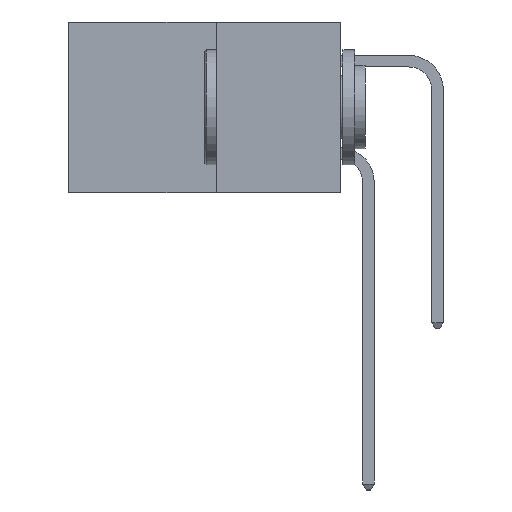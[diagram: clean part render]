
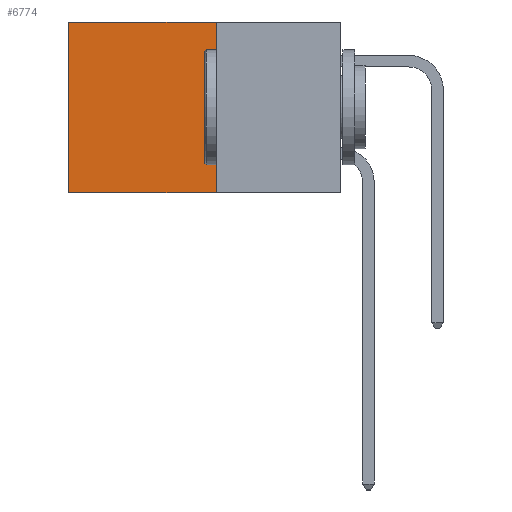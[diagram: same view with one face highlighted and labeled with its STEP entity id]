
A CAD part, left-side view. The second image highlights one B-rep face of the part: STEP entity #6774.
In plain terms, the highlighted planar face has unit normal (-1, 0, 0).
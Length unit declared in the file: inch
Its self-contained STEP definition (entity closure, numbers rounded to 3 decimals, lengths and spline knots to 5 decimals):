
#149 = VERTEX_POINT ( 'NONE', #4428 ) ;
#946 = EDGE_CURVE ( 'NONE', #6212, #1272, #7006, .T. ) ;
#1272 = VERTEX_POINT ( 'NONE', #6897 ) ;
#1538 = DIRECTION ( 'NONE',  ( 1., 0., 0. ) ) ;
#1558 = EDGE_LOOP ( 'NONE', ( #9436, #2102, #3152, #6438 ) ) ;
#2102 = ORIENTED_EDGE ( 'NONE', *, *, #9249, .F. ) ;
#2334 = EDGE_CURVE ( 'NONE', #6212, #7395, #4607, .T. ) ;
#2487 = VECTOR ( 'NONE', #5780, 39.37008 ) ;
#2665 = CARTESIAN_POINT ( 'NONE',  ( 0.277, 0.27, -0.37 ) ) ;
#3152 = ORIENTED_EDGE ( 'NONE', *, *, #946, .F. ) ;
#3175 = CARTESIAN_POINT ( 'NONE',  ( 0.277, 0.59, 0. ) ) ;
#3293 = AXIS2_PLACEMENT_3D ( 'NONE', #6301, #1538, #7115 ) ;
#3667 = LINE ( 'NONE', #8881, #7391 ) ;
#4302 = CARTESIAN_POINT ( 'NONE',  ( 0.277, 0.27, -0.37 ) ) ;
#4428 = CARTESIAN_POINT ( 'NONE',  ( 0.277, 0.59, -0.37 ) ) ;
#4607 = LINE ( 'NONE', #6411, #2487 ) ;
#4638 = VECTOR ( 'NONE', #9925, 39.37008 ) ;
#4718 = CARTESIAN_POINT ( 'NONE',  ( 0.277, 0.27, 0. ) ) ;
#5780 = DIRECTION ( 'NONE',  ( 0., 1., 0. ) ) ;
#6212 = VERTEX_POINT ( 'NONE', #4718 ) ;
#6301 = CARTESIAN_POINT ( 'NONE',  ( 0.277, 0.27, -0.37 ) ) ;
#6411 = CARTESIAN_POINT ( 'NONE',  ( 0.277, 0.27, 0. ) ) ;
#6438 = ORIENTED_EDGE ( 'NONE', *, *, #2334, .T. ) ;
#6458 = DIRECTION ( 'NONE',  ( 0., 0., -1. ) ) ;
#6774 = ADVANCED_FACE ( 'NONE', ( #9817 ), #9508, .F. ) ;
#6897 = CARTESIAN_POINT ( 'NONE',  ( 0.277, 0.27, -0.37 ) ) ;
#7006 = LINE ( 'NONE', #2665, #4638 ) ;
#7115 = DIRECTION ( 'NONE',  ( 0., 0., -1. ) ) ;
#7391 = VECTOR ( 'NONE', #6458, 39.37008 ) ;
#7395 = VERTEX_POINT ( 'NONE', #3175 ) ;
#8021 = VECTOR ( 'NONE', #9092, 39.37008 ) ;
#8881 = CARTESIAN_POINT ( 'NONE',  ( 0.277, 0.59, -0.37 ) ) ;
#9081 = EDGE_CURVE ( 'NONE', #7395, #149, #3667, .T. ) ;
#9092 = DIRECTION ( 'NONE',  ( 0., 1., 0. ) ) ;
#9249 = EDGE_CURVE ( 'NONE', #1272, #149, #10135, .T. ) ;
#9436 = ORIENTED_EDGE ( 'NONE', *, *, #9081, .T. ) ;
#9508 = PLANE ( 'NONE',  #3293 ) ;
#9817 = FACE_OUTER_BOUND ( 'NONE', #1558, .T. ) ;
#9925 = DIRECTION ( 'NONE',  ( 0., 0., -1. ) ) ;
#10135 = LINE ( 'NONE', #4302, #8021 ) ;
